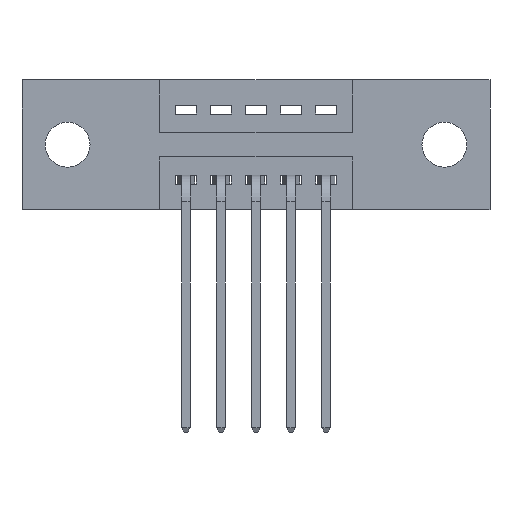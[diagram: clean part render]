
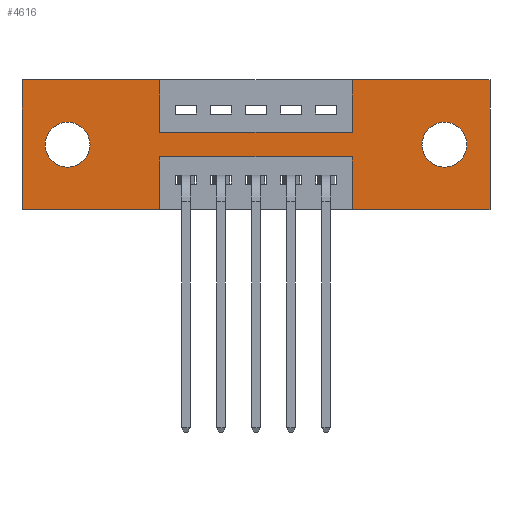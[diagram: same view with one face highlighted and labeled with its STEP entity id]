
A CAD part, front view. The second image highlights one B-rep face of the part: STEP entity #4616.
In plain terms, the highlighted planar face has unit normal (0, -1, 0).
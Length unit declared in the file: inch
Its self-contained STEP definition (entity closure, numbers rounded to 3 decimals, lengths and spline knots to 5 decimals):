
#11 = VECTOR ( 'NONE', #5054, 39.37008 ) ;
#17 = LINE ( 'NONE', #6406, #11 ) ;
#24 = CARTESIAN_POINT ( 'NONE',  ( 0.3925, 0., -0.37 ) ) ;
#85 = ORIENTED_EDGE ( 'NONE', *, *, #1421, .F. ) ;
#111 = DIRECTION ( 'NONE',  ( 1., 0., 0. ) ) ;
#159 = LINE ( 'NONE', #2178, #7201 ) ;
#198 = AXIS2_PLACEMENT_3D ( 'NONE', #3004, #7139, #2238 ) ;
#209 = EDGE_CURVE ( 'NONE', #3152, #1091, #159, .T. ) ;
#284 = EDGE_CURVE ( 'NONE', #6699, #5693, #3232, .T. ) ;
#305 = ORIENTED_EDGE ( 'NONE', *, *, #6824, .F. ) ;
#425 = ORIENTED_EDGE ( 'NONE', *, *, #209, .F. ) ;
#511 = DIRECTION ( 'NONE',  ( 0., 0., -1. ) ) ;
#514 = CARTESIAN_POINT ( 'NONE',  ( 1.205, 0., -0.121 ) ) ;
#659 = CARTESIAN_POINT ( 'NONE',  ( 0.13, 0., -0.185 ) ) ;
#687 = FACE_OUTER_BOUND ( 'NONE', #4724, .T. ) ;
#826 = CIRCLE ( 'NONE', #198, 0.064 ) ;
#865 = VERTEX_POINT ( 'NONE', #2460 ) ;
#875 = LINE ( 'NONE', #24, #4146 ) ;
#885 = LINE ( 'NONE', #7865, #7915 ) ;
#974 = DIRECTION ( 'NONE',  ( 0., -1., 0. ) ) ;
#1026 = VECTOR ( 'NONE', #4791, 39.37008 ) ;
#1031 = ORIENTED_EDGE ( 'NONE', *, *, #1500, .F. ) ;
#1091 = VERTEX_POINT ( 'NONE', #3585 ) ;
#1144 = VERTEX_POINT ( 'NONE', #1807 ) ;
#1187 = EDGE_LOOP ( 'NONE', ( #5744, #2691 ) ) ;
#1421 = EDGE_CURVE ( 'NONE', #4622, #2853, #6102, .T. ) ;
#1463 = DIRECTION ( 'NONE',  ( 0., 1., 0. ) ) ;
#1500 = EDGE_CURVE ( 'NONE', #1091, #6699, #885, .T. ) ;
#1547 = LINE ( 'NONE', #3588, #6765 ) ;
#1671 = EDGE_LOOP ( 'NONE', ( #7434, #7869 ) ) ;
#1715 = EDGE_CURVE ( 'NONE', #2693, #3098, #5989, .T. ) ;
#1774 = PLANE ( 'NONE',  #4166 ) ;
#1807 = CARTESIAN_POINT ( 'NONE',  ( 0.3925, 0., -0.22 ) ) ;
#1827 = ORIENTED_EDGE ( 'NONE', *, *, #6436, .F. ) ;
#1930 = CARTESIAN_POINT ( 'NONE',  ( 0., 0., -0.37 ) ) ;
#1966 = FACE_BOUND ( 'NONE', #1187, .T. ) ;
#2054 = CARTESIAN_POINT ( 'NONE',  ( 1.335, 0., 0. ) ) ;
#2142 = VECTOR ( 'NONE', #7082, 39.37008 ) ;
#2178 = CARTESIAN_POINT ( 'NONE',  ( 0.3925, 0., -0.15 ) ) ;
#2189 = CARTESIAN_POINT ( 'NONE',  ( 0., 0., 0. ) ) ;
#2229 = DIRECTION ( 'NONE',  ( 0., 0., 1. ) ) ;
#2238 = DIRECTION ( 'NONE',  ( 0., 0., -1. ) ) ;
#2254 = VERTEX_POINT ( 'NONE', #3581 ) ;
#2263 = FACE_BOUND ( 'NONE', #1671, .T. ) ;
#2298 = AXIS2_PLACEMENT_3D ( 'NONE', #5547, #1463, #2229 ) ;
#2350 = VECTOR ( 'NONE', #6254, 39.37008 ) ;
#2434 = DIRECTION ( 'NONE',  ( 0., 0., -1. ) ) ;
#2460 = CARTESIAN_POINT ( 'NONE',  ( 0.3925, 0., -0.37 ) ) ;
#2552 = LINE ( 'NONE', #7491, #3066 ) ;
#2637 = ORIENTED_EDGE ( 'NONE', *, *, #4843, .F. ) ;
#2638 = CARTESIAN_POINT ( 'NONE',  ( 0., 0., -0.37 ) ) ;
#2691 = ORIENTED_EDGE ( 'NONE', *, *, #6995, .T. ) ;
#2693 = VERTEX_POINT ( 'NONE', #8493 ) ;
#2822 = EDGE_CURVE ( 'NONE', #6097, #6521, #1547, .T. ) ;
#2853 = VERTEX_POINT ( 'NONE', #7856 ) ;
#2884 = ORIENTED_EDGE ( 'NONE', *, *, #6620, .F. ) ;
#2914 = CARTESIAN_POINT ( 'NONE',  ( 0.3925, 0., 0. ) ) ;
#3004 = CARTESIAN_POINT ( 'NONE',  ( 1.205, 0., -0.185 ) ) ;
#3066 = VECTOR ( 'NONE', #511, 39.37008 ) ;
#3098 = VERTEX_POINT ( 'NONE', #514 ) ;
#3152 = VERTEX_POINT ( 'NONE', #7276 ) ;
#3232 = LINE ( 'NONE', #4823, #1026 ) ;
#3294 = LINE ( 'NONE', #1930, #4032 ) ;
#3370 = ORIENTED_EDGE ( 'NONE', *, *, #8267, .F. ) ;
#3396 = CARTESIAN_POINT ( 'NONE',  ( 1.335, 0., -0.37 ) ) ;
#3581 = CARTESIAN_POINT ( 'NONE',  ( 0., 0., -0.37 ) ) ;
#3585 = CARTESIAN_POINT ( 'NONE',  ( 0.9425, 0., -0.15 ) ) ;
#3588 = CARTESIAN_POINT ( 'NONE',  ( 0., 0., 0. ) ) ;
#3734 = VERTEX_POINT ( 'NONE', #5818 ) ;
#3846 = ORIENTED_EDGE ( 'NONE', *, *, #6114, .F. ) ;
#4001 = VECTOR ( 'NONE', #4835, 39.37008 ) ;
#4032 = VECTOR ( 'NONE', #7480, 39.37008 ) ;
#4146 = VECTOR ( 'NONE', #5451, 39.37008 ) ;
#4166 = AXIS2_PLACEMENT_3D ( 'NONE', #8483, #974, #2434 ) ;
#4211 = ORIENTED_EDGE ( 'NONE', *, *, #5940, .F. ) ;
#4365 = CARTESIAN_POINT ( 'NONE',  ( 1.205, 0., -0.185 ) ) ;
#4428 = CARTESIAN_POINT ( 'NONE',  ( 0.9425, 0., -0.37 ) ) ;
#4616 = ADVANCED_FACE ( 'NONE', ( #2263, #1966, #687 ), #1774, .T. ) ;
#4622 = VERTEX_POINT ( 'NONE', #8453 ) ;
#4639 = EDGE_CURVE ( 'NONE', #3734, #5811, #8584, .T. ) ;
#4724 = EDGE_LOOP ( 'NONE', ( #4211, #305, #85, #1827, #2884, #5534, #1031, #425, #3370, #5690, #3846, #2637 ) ) ;
#4791 = DIRECTION ( 'NONE',  ( 1., 0., 0. ) ) ;
#4823 = CARTESIAN_POINT ( 'NONE',  ( 0., 0., 0. ) ) ;
#4835 = DIRECTION ( 'NONE',  ( 0., 0., -1. ) ) ;
#4843 = EDGE_CURVE ( 'NONE', #865, #2254, #7922, .T. ) ;
#5006 = LINE ( 'NONE', #6936, #2350 ) ;
#5054 = DIRECTION ( 'NONE',  ( -1., 0., 0. ) ) ;
#5073 = DIRECTION ( 'NONE',  ( 0., 0., -1. ) ) ;
#5421 = CIRCLE ( 'NONE', #2298, 0.064 ) ;
#5438 = DIRECTION ( 'NONE',  ( 0., 0., 1. ) ) ;
#5451 = DIRECTION ( 'NONE',  ( 0., 0., -1. ) ) ;
#5534 = ORIENTED_EDGE ( 'NONE', *, *, #284, .F. ) ;
#5547 = CARTESIAN_POINT ( 'NONE',  ( 0.13, 0., -0.185 ) ) ;
#5690 = ORIENTED_EDGE ( 'NONE', *, *, #2822, .F. ) ;
#5693 = VERTEX_POINT ( 'NONE', #2054 ) ;
#5744 = ORIENTED_EDGE ( 'NONE', *, *, #4639, .T. ) ;
#5811 = VERTEX_POINT ( 'NONE', #8327 ) ;
#5818 = CARTESIAN_POINT ( 'NONE',  ( 0.13, 0., -0.121 ) ) ;
#5831 = DIRECTION ( 'NONE',  ( 0., 1., 0. ) ) ;
#5940 = EDGE_CURVE ( 'NONE', #1144, #865, #875, .T. ) ;
#5989 = CIRCLE ( 'NONE', #6920, 0.064 ) ;
#6050 = LINE ( 'NONE', #8326, #4001 ) ;
#6097 = VERTEX_POINT ( 'NONE', #2189 ) ;
#6102 = LINE ( 'NONE', #4428, #2142 ) ;
#6106 = DIRECTION ( 'NONE',  ( 0., 1., 0. ) ) ;
#6114 = EDGE_CURVE ( 'NONE', #2254, #6097, #5006, .T. ) ;
#6254 = DIRECTION ( 'NONE',  ( 0., 0., 1. ) ) ;
#6328 = DIRECTION ( 'NONE',  ( 1., 0., 0. ) ) ;
#6406 = CARTESIAN_POINT ( 'NONE',  ( 0.3925, 0., -0.22 ) ) ;
#6436 = EDGE_CURVE ( 'NONE', #6902, #4622, #3294, .T. ) ;
#6521 = VERTEX_POINT ( 'NONE', #2914 ) ;
#6620 = EDGE_CURVE ( 'NONE', #5693, #6902, #2552, .T. ) ;
#6699 = VERTEX_POINT ( 'NONE', #7594 ) ;
#6765 = VECTOR ( 'NONE', #6328, 39.37008 ) ;
#6824 = EDGE_CURVE ( 'NONE', #2853, #1144, #17, .T. ) ;
#6902 = VERTEX_POINT ( 'NONE', #3396 ) ;
#6920 = AXIS2_PLACEMENT_3D ( 'NONE', #4365, #5831, #5073 ) ;
#6936 = CARTESIAN_POINT ( 'NONE',  ( 0., 0., 0. ) ) ;
#6995 = EDGE_CURVE ( 'NONE', #5811, #3734, #5421, .T. ) ;
#7082 = DIRECTION ( 'NONE',  ( 0., 0., 1. ) ) ;
#7139 = DIRECTION ( 'NONE',  ( 0., 1., 0. ) ) ;
#7201 = VECTOR ( 'NONE', #111, 39.37008 ) ;
#7231 = AXIS2_PLACEMENT_3D ( 'NONE', #659, #6106, #5438 ) ;
#7276 = CARTESIAN_POINT ( 'NONE',  ( 0.3925, 0., -0.15 ) ) ;
#7387 = DIRECTION ( 'NONE',  ( -1., 0., 0. ) ) ;
#7434 = ORIENTED_EDGE ( 'NONE', *, *, #8509, .T. ) ;
#7480 = DIRECTION ( 'NONE',  ( -1., 0., 0. ) ) ;
#7491 = CARTESIAN_POINT ( 'NONE',  ( 1.335, 0., 0. ) ) ;
#7594 = CARTESIAN_POINT ( 'NONE',  ( 0.9425, 0., 0. ) ) ;
#7709 = DIRECTION ( 'NONE',  ( 0., 0., 1. ) ) ;
#7819 = VECTOR ( 'NONE', #7387, 39.37008 ) ;
#7856 = CARTESIAN_POINT ( 'NONE',  ( 0.9425, 0., -0.22 ) ) ;
#7865 = CARTESIAN_POINT ( 'NONE',  ( 0.9425, 0., 0. ) ) ;
#7869 = ORIENTED_EDGE ( 'NONE', *, *, #1715, .T. ) ;
#7915 = VECTOR ( 'NONE', #7709, 39.37008 ) ;
#7922 = LINE ( 'NONE', #2638, #7819 ) ;
#8267 = EDGE_CURVE ( 'NONE', #6521, #3152, #6050, .T. ) ;
#8326 = CARTESIAN_POINT ( 'NONE',  ( 0.3925, 0., 0. ) ) ;
#8327 = CARTESIAN_POINT ( 'NONE',  ( 0.13, 0., -0.249 ) ) ;
#8453 = CARTESIAN_POINT ( 'NONE',  ( 0.9425, 0., -0.37 ) ) ;
#8483 = CARTESIAN_POINT ( 'NONE',  ( 0., 0., -0.37 ) ) ;
#8493 = CARTESIAN_POINT ( 'NONE',  ( 1.205, 0., -0.249 ) ) ;
#8509 = EDGE_CURVE ( 'NONE', #3098, #2693, #826, .T. ) ;
#8584 = CIRCLE ( 'NONE', #7231, 0.064 ) ;
